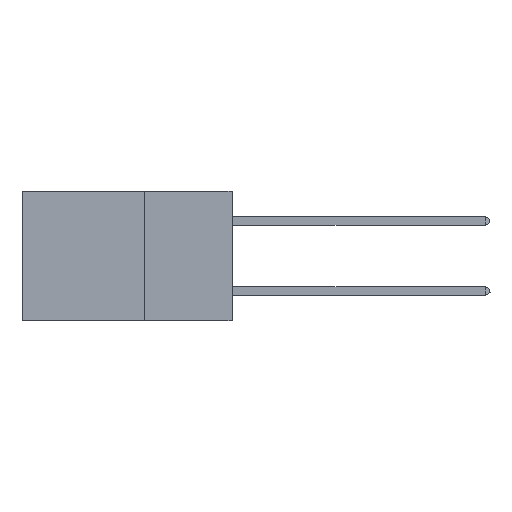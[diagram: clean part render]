
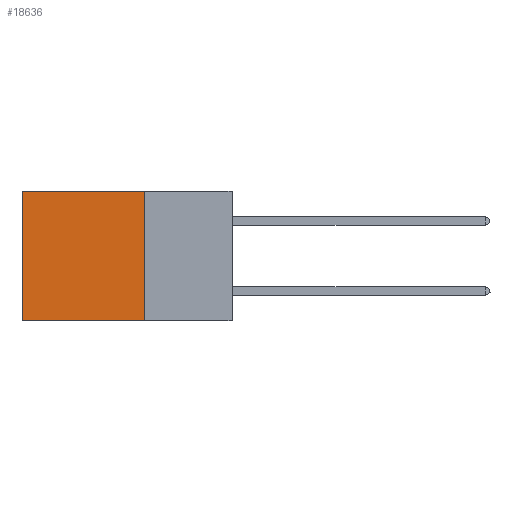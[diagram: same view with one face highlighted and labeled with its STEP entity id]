
A CAD part, left-side view. The second image highlights one B-rep face of the part: STEP entity #18636.
In plain terms, the highlighted planar face has unit normal (-1, 0, 0).
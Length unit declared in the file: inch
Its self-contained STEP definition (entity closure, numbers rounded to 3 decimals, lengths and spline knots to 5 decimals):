
#64 = CARTESIAN_POINT ( 'NONE',  ( 0.2875, 0.25, 0. ) ) ;
#616 = DIRECTION ( 'NONE',  ( 0., 0., -1. ) ) ;
#711 = CARTESIAN_POINT ( 'NONE',  ( 0.2875, 0.25, 0. ) ) ;
#1230 = ORIENTED_EDGE ( 'NONE', *, *, #10016, .F. ) ;
#1272 = LINE ( 'NONE', #6587, #9632 ) ;
#1415 = EDGE_LOOP ( 'NONE', ( #6860, #1230, #10494, #9823 ) ) ;
#3720 = LINE ( 'NONE', #4687, #11094 ) ;
#4049 = EDGE_CURVE ( 'NONE', #7087, #7812, #3720, .T. ) ;
#4412 = LINE ( 'NONE', #8856, #11526 ) ;
#4663 = PLANE ( 'NONE',  #14803 ) ;
#4687 = CARTESIAN_POINT ( 'NONE',  ( 0.2875, 0.25, 0. ) ) ;
#4746 = DIRECTION ( 'NONE',  ( 0., 1., 0. ) ) ;
#5031 = DIRECTION ( 'NONE',  ( 0., 0., -1. ) ) ;
#6587 = CARTESIAN_POINT ( 'NONE',  ( 0.2875, 0.6, 0. ) ) ;
#6860 = ORIENTED_EDGE ( 'NONE', *, *, #10881, .T. ) ;
#7087 = VERTEX_POINT ( 'NONE', #9844 ) ;
#7102 = EDGE_CURVE ( 'NONE', #7087, #14181, #14032, .T. ) ;
#7812 = VERTEX_POINT ( 'NONE', #18323 ) ;
#8350 = VECTOR ( 'NONE', #5031, 39.37008 ) ;
#8856 = CARTESIAN_POINT ( 'NONE',  ( 0.2875, 0.25, -0.37 ) ) ;
#9115 = DIRECTION ( 'NONE',  ( 0., 1., 0. ) ) ;
#9632 = VECTOR ( 'NONE', #616, 39.37008 ) ;
#9823 = ORIENTED_EDGE ( 'NONE', *, *, #4049, .T. ) ;
#9844 = CARTESIAN_POINT ( 'NONE',  ( 0.2875, 0.25, 0. ) ) ;
#10016 = EDGE_CURVE ( 'NONE', #14181, #13842, #4412, .T. ) ;
#10494 = ORIENTED_EDGE ( 'NONE', *, *, #7102, .F. ) ;
#10881 = EDGE_CURVE ( 'NONE', #7812, #13842, #1272, .T. ) ;
#11094 = VECTOR ( 'NONE', #4746, 39.37008 ) ;
#11526 = VECTOR ( 'NONE', #9115, 39.37008 ) ;
#13842 = VERTEX_POINT ( 'NONE', #15745 ) ;
#14032 = LINE ( 'NONE', #711, #8350 ) ;
#14181 = VERTEX_POINT ( 'NONE', #15051 ) ;
#14803 = AXIS2_PLACEMENT_3D ( 'NONE', #64, #15407, #18223 ) ;
#15051 = CARTESIAN_POINT ( 'NONE',  ( 0.2875, 0.25, -0.37 ) ) ;
#15407 = DIRECTION ( 'NONE',  ( 1., 0., 0. ) ) ;
#15745 = CARTESIAN_POINT ( 'NONE',  ( 0.2875, 0.6, -0.37 ) ) ;
#17436 = FACE_OUTER_BOUND ( 'NONE', #1415, .T. ) ;
#18223 = DIRECTION ( 'NONE',  ( 0., 0., -1. ) ) ;
#18323 = CARTESIAN_POINT ( 'NONE',  ( 0.2875, 0.6, 0. ) ) ;
#18636 = ADVANCED_FACE ( 'NONE', ( #17436 ), #4663, .F. ) ;
